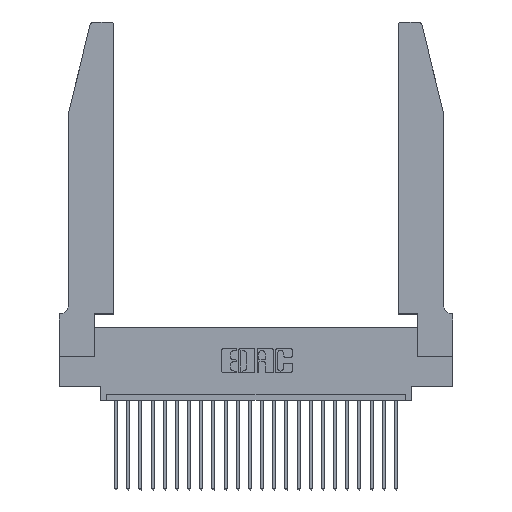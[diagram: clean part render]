
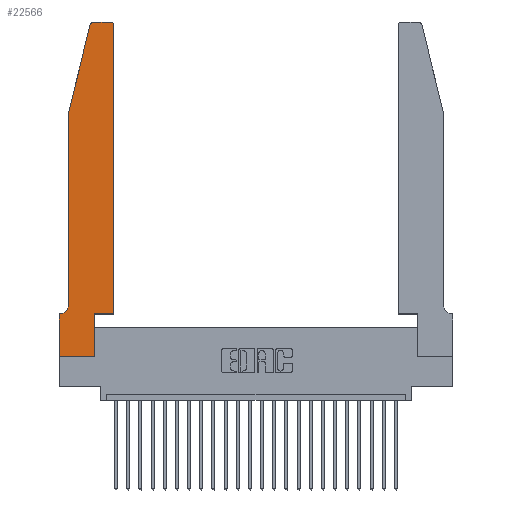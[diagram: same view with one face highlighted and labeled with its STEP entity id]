
A CAD part, top view. The second image highlights one B-rep face of the part: STEP entity #22566.
In plain terms, the highlighted planar face has unit normal (0, 0, 1).
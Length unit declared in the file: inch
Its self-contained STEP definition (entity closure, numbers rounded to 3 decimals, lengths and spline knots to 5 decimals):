
#341 = VECTOR ( 'NONE', #7812, 39.37008 ) ;
#718 = CIRCLE ( 'NONE', #4871, 0.07 ) ;
#1137 = CARTESIAN_POINT ( 'NONE',  ( 0.0755, 2., 0.37 ) ) ;
#1396 = DIRECTION ( 'NONE',  ( -0.239, -0.971, 0. ) ) ;
#1535 = CARTESIAN_POINT ( 'NONE',  ( 0.2865, 0.35, 0.37 ) ) ;
#1889 = VERTEX_POINT ( 'NONE', #17323 ) ;
#2349 = VERTEX_POINT ( 'NONE', #14427 ) ;
#2448 = VERTEX_POINT ( 'NONE', #1137 ) ;
#2524 = EDGE_CURVE ( 'NONE', #2448, #1889, #8591, .T. ) ;
#2556 = EDGE_LOOP ( 'NONE', ( #7829, #9687, #3616, #5410, #12453, #8036, #24052, #17600, #12751, #13877, #8788, #24162 ) ) ;
#2831 = AXIS2_PLACEMENT_3D ( 'NONE', #4782, #6686, #12763 ) ;
#2958 = EDGE_CURVE ( 'NONE', #19137, #8754, #8577, .T. ) ;
#3058 = CARTESIAN_POINT ( 'NONE',  ( 0., 0.35, 0.37 ) ) ;
#3280 = EDGE_CURVE ( 'NONE', #7491, #7079, #24572, .T. ) ;
#3616 = ORIENTED_EDGE ( 'NONE', *, *, #17245, .T. ) ;
#4782 = CARTESIAN_POINT ( 'NONE',  ( 0.4205, 2.72, 0.37 ) ) ;
#4871 = AXIS2_PLACEMENT_3D ( 'NONE', #20105, #12142, #24041 ) ;
#5170 = DIRECTION ( 'NONE',  ( 1., 0., 0. ) ) ;
#5214 = PLANE ( 'NONE',  #14072 ) ;
#5410 = ORIENTED_EDGE ( 'NONE', *, *, #2524, .T. ) ;
#5944 = CARTESIAN_POINT ( 'NONE',  ( 0., 0.35, 0.37 ) ) ;
#6154 = CARTESIAN_POINT ( 'NONE',  ( 0.4505, 2.72, 0.37 ) ) ;
#6227 = CARTESIAN_POINT ( 'NONE',  ( 0.25487, 2.72718, 0.37 ) ) ;
#6412 = CARTESIAN_POINT ( 'NONE',  ( 0.0755, 0.35, 0.37 ) ) ;
#6545 = VERTEX_POINT ( 'NONE', #5944 ) ;
#6686 = DIRECTION ( 'NONE',  ( 0., 0., 1. ) ) ;
#6748 = VERTEX_POINT ( 'NONE', #10014 ) ;
#7079 = VERTEX_POINT ( 'NONE', #24141 ) ;
#7344 = LINE ( 'NONE', #8300, #12563 ) ;
#7491 = VERTEX_POINT ( 'NONE', #6154 ) ;
#7812 = DIRECTION ( 'NONE',  ( 0., -1., 0. ) ) ;
#7816 = CIRCLE ( 'NONE', #16946, 0.03 ) ;
#7829 = ORIENTED_EDGE ( 'NONE', *, *, #21772, .T. ) ;
#8036 = ORIENTED_EDGE ( 'NONE', *, *, #15075, .T. ) ;
#8129 = EDGE_CURVE ( 'NONE', #1889, #2349, #718, .T. ) ;
#8135 = VERTEX_POINT ( 'NONE', #16179 ) ;
#8284 = CARTESIAN_POINT ( 'NONE',  ( 0.4505, 0.35, 0.37 ) ) ;
#8296 = EDGE_CURVE ( 'NONE', #16066, #19137, #18778, .T. ) ;
#8300 = CARTESIAN_POINT ( 'NONE',  ( 0., 0., 0.37 ) ) ;
#8577 = LINE ( 'NONE', #11001, #23547 ) ;
#8591 = LINE ( 'NONE', #8738, #15014 ) ;
#8686 = EDGE_CURVE ( 'NONE', #6545, #8135, #23657, .T. ) ;
#8738 = CARTESIAN_POINT ( 'NONE',  ( 0.0755, 2., 0.37 ) ) ;
#8754 = VERTEX_POINT ( 'NONE', #8284 ) ;
#8788 = ORIENTED_EDGE ( 'NONE', *, *, #12987, .T. ) ;
#9687 = ORIENTED_EDGE ( 'NONE', *, *, #13981, .T. ) ;
#10014 = CARTESIAN_POINT ( 'NONE',  ( 0.284, 2.75, 0.37 ) ) ;
#10211 = VECTOR ( 'NONE', #23148, 39.37008 ) ;
#10500 = CARTESIAN_POINT ( 'NONE',  ( 0., 0., 0.37 ) ) ;
#10659 = DIRECTION ( 'NONE',  ( -1., 0., 0. ) ) ;
#10696 = CARTESIAN_POINT ( 'NONE',  ( 0.0755, 2., 0.37 ) ) ;
#11001 = CARTESIAN_POINT ( 'NONE',  ( 0.4505, 0.35, 0.37 ) ) ;
#11031 = DIRECTION ( 'NONE',  ( -1., 0., 0. ) ) ;
#11451 = CARTESIAN_POINT ( 'NONE',  ( 0.2865, 0., 0.37 ) ) ;
#12142 = DIRECTION ( 'NONE',  ( 0., 0., -1. ) ) ;
#12453 = ORIENTED_EDGE ( 'NONE', *, *, #8129, .T. ) ;
#12563 = VECTOR ( 'NONE', #21989, 39.37008 ) ;
#12751 = ORIENTED_EDGE ( 'NONE', *, *, #8296, .T. ) ;
#12754 = DIRECTION ( 'NONE',  ( 0., -1., 0. ) ) ;
#12763 = DIRECTION ( 'NONE',  ( 1., 0., 0. ) ) ;
#12987 = EDGE_CURVE ( 'NONE', #8754, #7491, #19213, .T. ) ;
#13868 = DIRECTION ( 'NONE',  ( 0., 1., 0. ) ) ;
#13877 = ORIENTED_EDGE ( 'NONE', *, *, #2958, .T. ) ;
#13981 = EDGE_CURVE ( 'NONE', #6748, #22301, #7816, .T. ) ;
#14072 = AXIS2_PLACEMENT_3D ( 'NONE', #3058, #20715, #18567 ) ;
#14427 = CARTESIAN_POINT ( 'NONE',  ( 0.0055, 0.35, 0.37 ) ) ;
#14757 = CARTESIAN_POINT ( 'NONE',  ( 0.2605, 2.75, 0.37 ) ) ;
#15014 = VECTOR ( 'NONE', #12754, 39.37008 ) ;
#15075 = EDGE_CURVE ( 'NONE', #2349, #6545, #16367, .T. ) ;
#15583 = CARTESIAN_POINT ( 'NONE',  ( 0.2865, 0.35, 0.37 ) ) ;
#15745 = VECTOR ( 'NONE', #11031, 39.37008 ) ;
#15762 = CARTESIAN_POINT ( 'NONE',  ( 0.4505, 0.35, 0.37 ) ) ;
#16066 = VERTEX_POINT ( 'NONE', #11451 ) ;
#16179 = CARTESIAN_POINT ( 'NONE',  ( 0., 0., 0.37 ) ) ;
#16367 = LINE ( 'NONE', #6412, #15745 ) ;
#16946 = AXIS2_PLACEMENT_3D ( 'NONE', #24895, #20712, #18886 ) ;
#17245 = EDGE_CURVE ( 'NONE', #22301, #2448, #18430, .T. ) ;
#17323 = CARTESIAN_POINT ( 'NONE',  ( 0.0755, 0.42, 0.37 ) ) ;
#17600 = ORIENTED_EDGE ( 'NONE', *, *, #18231, .T. ) ;
#18231 = EDGE_CURVE ( 'NONE', #8135, #16066, #7344, .T. ) ;
#18430 = LINE ( 'NONE', #10696, #23614 ) ;
#18567 = DIRECTION ( 'NONE',  ( 1., 0., 0. ) ) ;
#18778 = LINE ( 'NONE', #1535, #10211 ) ;
#18886 = DIRECTION ( 'NONE',  ( 1., 0., 0. ) ) ;
#19137 = VERTEX_POINT ( 'NONE', #15583 ) ;
#19213 = LINE ( 'NONE', #15762, #21679 ) ;
#20105 = CARTESIAN_POINT ( 'NONE',  ( 0.0055, 0.42, 0.37 ) ) ;
#20712 = DIRECTION ( 'NONE',  ( 0., 0., 1. ) ) ;
#20715 = DIRECTION ( 'NONE',  ( 0., 0., 1. ) ) ;
#21679 = VECTOR ( 'NONE', #13868, 39.37008 ) ;
#21772 = EDGE_CURVE ( 'NONE', #7079, #6748, #23406, .T. ) ;
#21989 = DIRECTION ( 'NONE',  ( 1., 0., 0. ) ) ;
#22301 = VERTEX_POINT ( 'NONE', #6227 ) ;
#22474 = FACE_OUTER_BOUND ( 'NONE', #2556, .T. ) ;
#22566 = ADVANCED_FACE ( 'NONE', ( #22474 ), #5214, .T. ) ;
#23148 = DIRECTION ( 'NONE',  ( 0., 1., 0. ) ) ;
#23406 = LINE ( 'NONE', #14757, #24021 ) ;
#23547 = VECTOR ( 'NONE', #5170, 39.37008 ) ;
#23614 = VECTOR ( 'NONE', #1396, 39.37008 ) ;
#23657 = LINE ( 'NONE', #10500, #341 ) ;
#24021 = VECTOR ( 'NONE', #10659, 39.37008 ) ;
#24041 = DIRECTION ( 'NONE',  ( -1., 0., 0. ) ) ;
#24052 = ORIENTED_EDGE ( 'NONE', *, *, #8686, .T. ) ;
#24141 = CARTESIAN_POINT ( 'NONE',  ( 0.4205, 2.75, 0.37 ) ) ;
#24162 = ORIENTED_EDGE ( 'NONE', *, *, #3280, .T. ) ;
#24572 = CIRCLE ( 'NONE', #2831, 0.03 ) ;
#24895 = CARTESIAN_POINT ( 'NONE',  ( 0.284, 2.72, 0.37 ) ) ;
